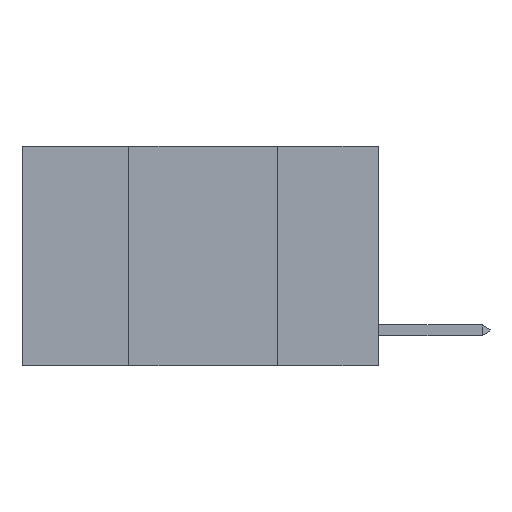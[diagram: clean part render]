
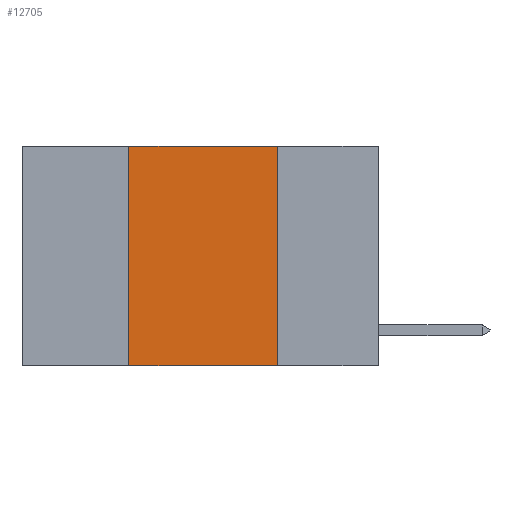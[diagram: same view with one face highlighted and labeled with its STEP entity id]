
A CAD part, left-side view. The second image highlights one B-rep face of the part: STEP entity #12705.
In plain terms, the highlighted planar face has unit normal (-1, 0, 0).
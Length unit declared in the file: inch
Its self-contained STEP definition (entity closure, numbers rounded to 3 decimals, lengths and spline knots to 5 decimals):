
#359 = VERTEX_POINT ( 'NONE', #7983 ) ;
#695 = CARTESIAN_POINT ( 'NONE',  ( 0., 0.42, 0. ) ) ;
#739 = CARTESIAN_POINT ( 'NONE',  ( 0., 0.17, 0. ) ) ;
#1013 = CARTESIAN_POINT ( 'NONE',  ( 0., 0.6, -0.37 ) ) ;
#1828 = ORIENTED_EDGE ( 'NONE', *, *, #5072, .F. ) ;
#1846 = VECTOR ( 'NONE', #7557, 39.37008 ) ;
#2136 = CARTESIAN_POINT ( 'NONE',  ( 0., 0.17, 0. ) ) ;
#2199 = EDGE_CURVE ( 'NONE', #359, #11787, #10940, .T. ) ;
#2356 = VECTOR ( 'NONE', #4411, 39.37008 ) ;
#2454 = VERTEX_POINT ( 'NONE', #695 ) ;
#3613 = CARTESIAN_POINT ( 'NONE',  ( 0., 0.42, 0. ) ) ;
#3696 = DIRECTION ( 'NONE',  ( 0., 0., -1. ) ) ;
#3816 = EDGE_LOOP ( 'NONE', ( #7132, #1828, #12883, #6007 ) ) ;
#4411 = DIRECTION ( 'NONE',  ( 0., -1., 0. ) ) ;
#4640 = DIRECTION ( 'NONE',  ( 1., 0., 0. ) ) ;
#4687 = EDGE_CURVE ( 'NONE', #12573, #11787, #8157, .T. ) ;
#5072 = EDGE_CURVE ( 'NONE', #2454, #12573, #12090, .T. ) ;
#5197 = EDGE_CURVE ( 'NONE', #359, #2454, #12377, .T. ) ;
#5357 = AXIS2_PLACEMENT_3D ( 'NONE', #11101, #4640, #3696 ) ;
#5537 = FACE_OUTER_BOUND ( 'NONE', #3816, .T. ) ;
#6007 = ORIENTED_EDGE ( 'NONE', *, *, #2199, .T. ) ;
#6880 = DIRECTION ( 'NONE',  ( 0., 0., 1. ) ) ;
#7132 = ORIENTED_EDGE ( 'NONE', *, *, #4687, .F. ) ;
#7557 = DIRECTION ( 'NONE',  ( 0., -1., 0. ) ) ;
#7597 = VECTOR ( 'NONE', #8438, 39.37008 ) ;
#7983 = CARTESIAN_POINT ( 'NONE',  ( 0., 0.42, -0.37 ) ) ;
#8121 = CARTESIAN_POINT ( 'NONE',  ( 0., 0.17, -0.37 ) ) ;
#8157 = LINE ( 'NONE', #739, #7597 ) ;
#8438 = DIRECTION ( 'NONE',  ( 0., 0., -1. ) ) ;
#9845 = CARTESIAN_POINT ( 'NONE',  ( 0., 0.6, 0. ) ) ;
#10115 = PLANE ( 'NONE',  #5357 ) ;
#10940 = LINE ( 'NONE', #1013, #1846 ) ;
#11101 = CARTESIAN_POINT ( 'NONE',  ( 0., 0.6, 0. ) ) ;
#11787 = VERTEX_POINT ( 'NONE', #8121 ) ;
#11918 = VECTOR ( 'NONE', #6880, 39.37008 ) ;
#12090 = LINE ( 'NONE', #9845, #2356 ) ;
#12377 = LINE ( 'NONE', #3613, #11918 ) ;
#12573 = VERTEX_POINT ( 'NONE', #2136 ) ;
#12705 = ADVANCED_FACE ( 'NONE', ( #5537 ), #10115, .F. ) ;
#12883 = ORIENTED_EDGE ( 'NONE', *, *, #5197, .F. ) ;
